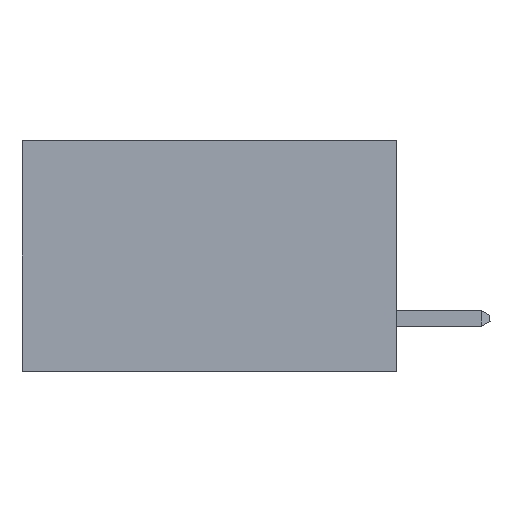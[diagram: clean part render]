
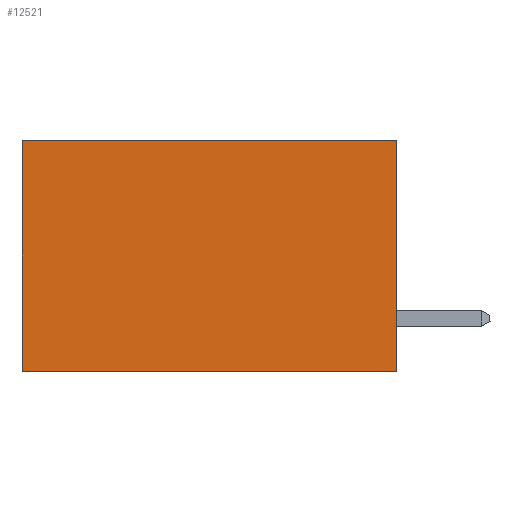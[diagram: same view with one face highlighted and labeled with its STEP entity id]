
A CAD part, left-side view. The second image highlights one B-rep face of the part: STEP entity #12521.
In plain terms, the highlighted planar face has unit normal (-1, 0, 0).
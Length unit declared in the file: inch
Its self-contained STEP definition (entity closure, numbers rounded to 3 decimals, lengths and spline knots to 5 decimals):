
#37 = PLANE ( 'NONE',  #7931 ) ;
#2249 = DIRECTION ( 'NONE',  ( 0., 0., -1. ) ) ;
#2250 = VERTEX_POINT ( 'NONE', #7466 ) ;
#2356 = LINE ( 'NONE', #5728, #8314 ) ;
#2572 = DIRECTION ( 'NONE',  ( 0., 1., 0. ) ) ;
#3369 = EDGE_CURVE ( 'NONE', #8677, #2250, #3915, .T. ) ;
#3915 = LINE ( 'NONE', #7460, #9154 ) ;
#4349 = CARTESIAN_POINT ( 'NONE',  ( 0.298, 0., 0. ) ) ;
#5061 = EDGE_CURVE ( 'NONE', #9400, #8677, #2356, .T. ) ;
#5166 = CARTESIAN_POINT ( 'NONE',  ( 0.298, 0.6, 0. ) ) ;
#5223 = EDGE_CURVE ( 'NONE', #9400, #6809, #6002, .T. ) ;
#5728 = CARTESIAN_POINT ( 'NONE',  ( 0.298, 0., 0. ) ) ;
#5750 = ORIENTED_EDGE ( 'NONE', *, *, #7774, .T. ) ;
#6002 = LINE ( 'NONE', #6503, #8470 ) ;
#6105 = ORIENTED_EDGE ( 'NONE', *, *, #5061, .F. ) ;
#6457 = ORIENTED_EDGE ( 'NONE', *, *, #5223, .T. ) ;
#6503 = CARTESIAN_POINT ( 'NONE',  ( 0.298, 0., 0. ) ) ;
#6598 = CARTESIAN_POINT ( 'NONE',  ( 0.298, 0.6, 0. ) ) ;
#6809 = VERTEX_POINT ( 'NONE', #6598 ) ;
#7460 = CARTESIAN_POINT ( 'NONE',  ( 0.298, 0., -0.37 ) ) ;
#7466 = CARTESIAN_POINT ( 'NONE',  ( 0.298, 0.6, -0.37 ) ) ;
#7774 = EDGE_CURVE ( 'NONE', #6809, #2250, #8606, .T. ) ;
#7931 = AXIS2_PLACEMENT_3D ( 'NONE', #4349, #8569, #2249 ) ;
#8027 = EDGE_LOOP ( 'NONE', ( #5750, #11052, #6105, #6457 ) ) ;
#8314 = VECTOR ( 'NONE', #11838, 39.37008 ) ;
#8470 = VECTOR ( 'NONE', #2572, 39.37008 ) ;
#8569 = DIRECTION ( 'NONE',  ( 1., 0., 0. ) ) ;
#8606 = LINE ( 'NONE', #5166, #11088 ) ;
#8676 = CARTESIAN_POINT ( 'NONE',  ( 0.298, 0., 0. ) ) ;
#8677 = VERTEX_POINT ( 'NONE', #11834 ) ;
#9154 = VECTOR ( 'NONE', #10689, 39.37008 ) ;
#9400 = VERTEX_POINT ( 'NONE', #8676 ) ;
#10689 = DIRECTION ( 'NONE',  ( 0., 1., 0. ) ) ;
#11052 = ORIENTED_EDGE ( 'NONE', *, *, #3369, .F. ) ;
#11088 = VECTOR ( 'NONE', #12549, 39.37008 ) ;
#11424 = FACE_OUTER_BOUND ( 'NONE', #8027, .T. ) ;
#11834 = CARTESIAN_POINT ( 'NONE',  ( 0.298, 0., -0.37 ) ) ;
#11838 = DIRECTION ( 'NONE',  ( 0., 0., -1. ) ) ;
#12521 = ADVANCED_FACE ( 'NONE', ( #11424 ), #37, .F. ) ;
#12549 = DIRECTION ( 'NONE',  ( 0., 0., -1. ) ) ;
